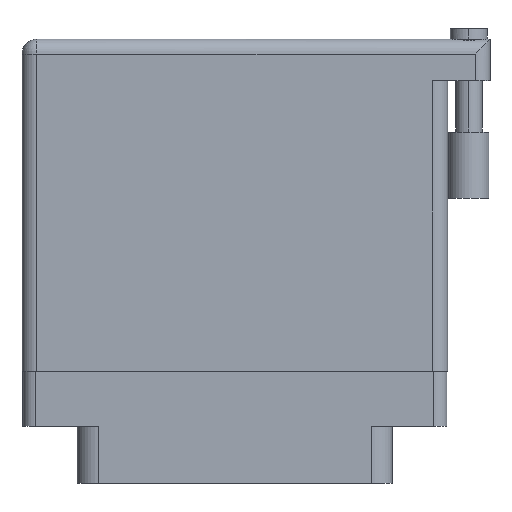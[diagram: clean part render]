
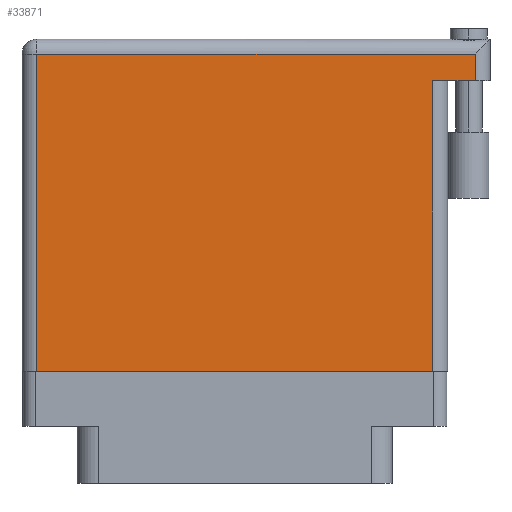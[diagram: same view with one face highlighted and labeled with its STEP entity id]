
A CAD part, front view. The second image highlights one B-rep face of the part: STEP entity #33871.
In plain terms, the highlighted face is planar.
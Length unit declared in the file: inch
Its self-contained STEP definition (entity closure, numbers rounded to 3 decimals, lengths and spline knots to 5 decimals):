
#849 = DIRECTION ( 'NONE',  ( -1., 0., 0. ) ) ;
#2065 = DIRECTION ( 'NONE',  ( 0., -1., 0. ) ) ;
#2854 = ORIENTED_EDGE ( 'NONE', *, *, #13003, .T. ) ;
#3451 = VERTEX_POINT ( 'NONE', #11399 ) ;
#4970 = EDGE_CURVE ( 'NONE', #31172, #27115, #37678, .T. ) ;
#5273 = VERTEX_POINT ( 'NONE', #23521 ) ;
#5578 = ORIENTED_EDGE ( 'NONE', *, *, #4970, .T. ) ;
#5884 = ORIENTED_EDGE ( 'NONE', *, *, #14920, .T. ) ;
#8162 = DIRECTION ( 'NONE',  ( 0., 0., -1. ) ) ;
#8668 = PLANE ( 'NONE',  #19280 ) ;
#9561 = DIRECTION ( 'NONE',  ( 0., 1., 0. ) ) ;
#10866 = VERTEX_POINT ( 'NONE', #32737 ) ;
#11399 = CARTESIAN_POINT ( 'NONE',  ( 2.138, 1.369, 0. ) ) ;
#13003 = EDGE_CURVE ( 'NONE', #5273, #30124, #25988, .T. ) ;
#13082 = VECTOR ( 'NONE', #9561, 39.37008 ) ;
#14815 = EDGE_LOOP ( 'NONE', ( #2854, #21952, #27082, #32484, #5578, #5884 ) ) ;
#14920 = EDGE_CURVE ( 'NONE', #27115, #5273, #15531, .T. ) ;
#15427 = EDGE_CURVE ( 'NONE', #3451, #10866, #37989, .T. ) ;
#15531 = LINE ( 'NONE', #34865, #38020 ) ;
#18482 = VECTOR ( 'NONE', #21125, 39.37008 ) ;
#18837 = CARTESIAN_POINT ( 'NONE',  ( 0., 1.496, 0. ) ) ;
#19280 = AXIS2_PLACEMENT_3D ( 'NONE', #32308, #8162, #29144 ) ;
#19427 = VECTOR ( 'NONE', #849, 39.37008 ) ;
#20632 = DIRECTION ( 'NONE',  ( -1., 0., 0. ) ) ;
#20881 = CARTESIAN_POINT ( 'NONE',  ( 2.138, 1.566, 0. ) ) ;
#21125 = DIRECTION ( 'NONE',  ( 0., 1., 0. ) ) ;
#21797 = CARTESIAN_POINT ( 'NONE',  ( 1.938, 0., 0. ) ) ;
#21952 = ORIENTED_EDGE ( 'NONE', *, *, #34816, .T. ) ;
#21989 = LINE ( 'NONE', #27529, #13082 ) ;
#23500 = EDGE_CURVE ( 'NONE', #3451, #31172, #38150, .T. ) ;
#23521 = CARTESIAN_POINT ( 'NONE',  ( 0.07, 0., 0. ) ) ;
#25988 = LINE ( 'NONE', #35689, #27859 ) ;
#27082 = ORIENTED_EDGE ( 'NONE', *, *, #15427, .F. ) ;
#27115 = VERTEX_POINT ( 'NONE', #32329 ) ;
#27529 = CARTESIAN_POINT ( 'NONE',  ( 1.938, 1.369, 0. ) ) ;
#27859 = VECTOR ( 'NONE', #33557, 39.37008 ) ;
#28655 = VECTOR ( 'NONE', #20632, 39.37008 ) ;
#29144 = DIRECTION ( 'NONE',  ( -1., 0., 0. ) ) ;
#29707 = CARTESIAN_POINT ( 'NONE',  ( 2.138, 1.496, 0. ) ) ;
#30124 = VERTEX_POINT ( 'NONE', #21797 ) ;
#31172 = VERTEX_POINT ( 'NONE', #29707 ) ;
#32308 = CARTESIAN_POINT ( 'NONE',  ( 0., 1.566, 0. ) ) ;
#32329 = CARTESIAN_POINT ( 'NONE',  ( 0.07, 1.496, 0. ) ) ;
#32484 = ORIENTED_EDGE ( 'NONE', *, *, #23500, .T. ) ;
#32737 = CARTESIAN_POINT ( 'NONE',  ( 1.938, 1.369, 0. ) ) ;
#33056 = CARTESIAN_POINT ( 'NONE',  ( 2.208, 1.369, 0. ) ) ;
#33557 = DIRECTION ( 'NONE',  ( 1., 0., 0. ) ) ;
#33871 = ADVANCED_FACE ( 'NONE', ( #35676 ), #8668, .F. ) ;
#34816 = EDGE_CURVE ( 'NONE', #30124, #10866, #21989, .T. ) ;
#34865 = CARTESIAN_POINT ( 'NONE',  ( 0.07, 0., 0. ) ) ;
#35676 = FACE_OUTER_BOUND ( 'NONE', #14815, .T. ) ;
#35689 = CARTESIAN_POINT ( 'NONE',  ( 0., 0., 0. ) ) ;
#37678 = LINE ( 'NONE', #18837, #19427 ) ;
#37989 = LINE ( 'NONE', #33056, #28655 ) ;
#38020 = VECTOR ( 'NONE', #2065, 39.37008 ) ;
#38150 = LINE ( 'NONE', #20881, #18482 ) ;
